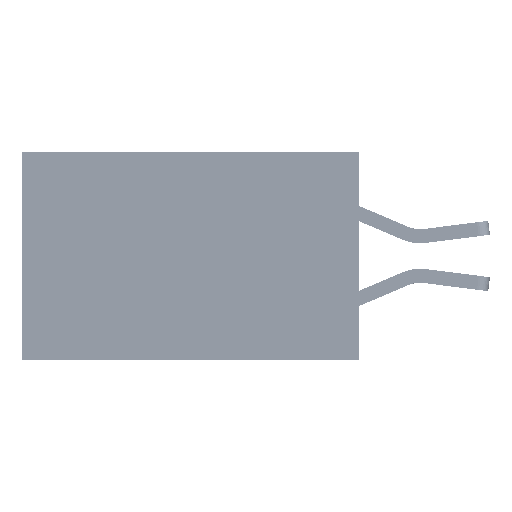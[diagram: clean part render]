
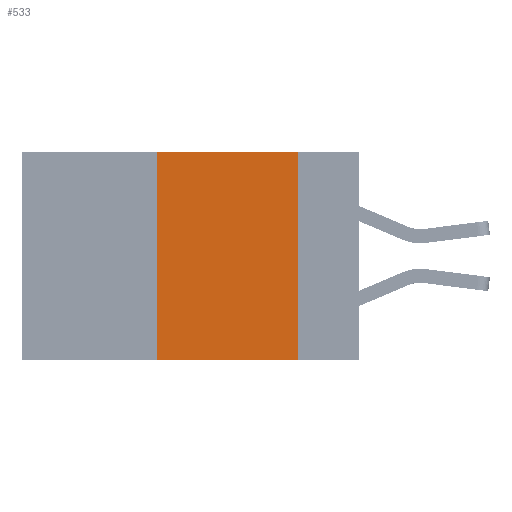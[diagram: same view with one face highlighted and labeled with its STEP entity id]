
A CAD part, left-side view. The second image highlights one B-rep face of the part: STEP entity #533.
In plain terms, the highlighted planar face has unit normal (-1, 0, 0).
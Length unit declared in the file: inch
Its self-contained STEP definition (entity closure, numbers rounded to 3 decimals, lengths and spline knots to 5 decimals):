
#132 = CARTESIAN_POINT ( 'NONE',  ( 0., 0.36, 0. ) ) ;
#533 = ADVANCED_FACE ( 'NONE', ( #29717 ), #39120, .F. ) ;
#944 = DIRECTION ( 'NONE',  ( 0., 0., -1. ) ) ;
#4206 = AXIS2_PLACEMENT_3D ( 'NONE', #42829, #23504, #11924 ) ;
#4955 = LINE ( 'NONE', #43015, #38428 ) ;
#5311 = VECTOR ( 'NONE', #40628, 39.37008 ) ;
#7320 = DIRECTION ( 'NONE',  ( 0., 0., 1. ) ) ;
#11924 = DIRECTION ( 'NONE',  ( 0., 0., -1. ) ) ;
#12954 = VECTOR ( 'NONE', #944, 39.37008 ) ;
#13779 = VERTEX_POINT ( 'NONE', #31943 ) ;
#14165 = LINE ( 'NONE', #43434, #12954 ) ;
#21378 = LINE ( 'NONE', #26709, #23194 ) ;
#21394 = VERTEX_POINT ( 'NONE', #132 ) ;
#21670 = CARTESIAN_POINT ( 'NONE',  ( 0., 0.6, -0.37 ) ) ;
#23194 = VECTOR ( 'NONE', #7320, 39.37008 ) ;
#23504 = DIRECTION ( 'NONE',  ( 1., 0., 0. ) ) ;
#26709 = CARTESIAN_POINT ( 'NONE',  ( 0., 0.36, 0. ) ) ;
#26881 = ORIENTED_EDGE ( 'NONE', *, *, #31951, .F. ) ;
#29024 = VERTEX_POINT ( 'NONE', #29614 ) ;
#29614 = CARTESIAN_POINT ( 'NONE',  ( 0., 0.11, 0. ) ) ;
#29717 = FACE_OUTER_BOUND ( 'NONE', #30821, .T. ) ;
#30821 = EDGE_LOOP ( 'NONE', ( #26881, #43448, #31822, #36231 ) ) ;
#31822 = ORIENTED_EDGE ( 'NONE', *, *, #36650, .F. ) ;
#31943 = CARTESIAN_POINT ( 'NONE',  ( 0., 0.36, -0.37 ) ) ;
#31951 = EDGE_CURVE ( 'NONE', #29024, #45851, #14165, .T. ) ;
#32104 = LINE ( 'NONE', #21670, #5311 ) ;
#36231 = ORIENTED_EDGE ( 'NONE', *, *, #47848, .T. ) ;
#36650 = EDGE_CURVE ( 'NONE', #13779, #21394, #21378, .T. ) ;
#38428 = VECTOR ( 'NONE', #50329, 39.37008 ) ;
#39120 = PLANE ( 'NONE',  #4206 ) ;
#40628 = DIRECTION ( 'NONE',  ( 0., -1., 0. ) ) ;
#41880 = EDGE_CURVE ( 'NONE', #21394, #29024, #4955, .T. ) ;
#42829 = CARTESIAN_POINT ( 'NONE',  ( 0., 0.6, 0. ) ) ;
#43015 = CARTESIAN_POINT ( 'NONE',  ( 0., 0.6, 0. ) ) ;
#43404 = CARTESIAN_POINT ( 'NONE',  ( 0., 0.11, -0.37 ) ) ;
#43434 = CARTESIAN_POINT ( 'NONE',  ( 0., 0.11, 0. ) ) ;
#43448 = ORIENTED_EDGE ( 'NONE', *, *, #41880, .F. ) ;
#45851 = VERTEX_POINT ( 'NONE', #43404 ) ;
#47848 = EDGE_CURVE ( 'NONE', #13779, #45851, #32104, .T. ) ;
#50329 = DIRECTION ( 'NONE',  ( 0., -1., 0. ) ) ;
